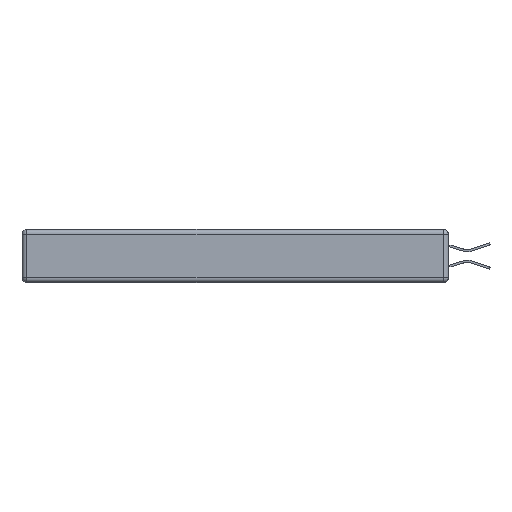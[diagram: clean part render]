
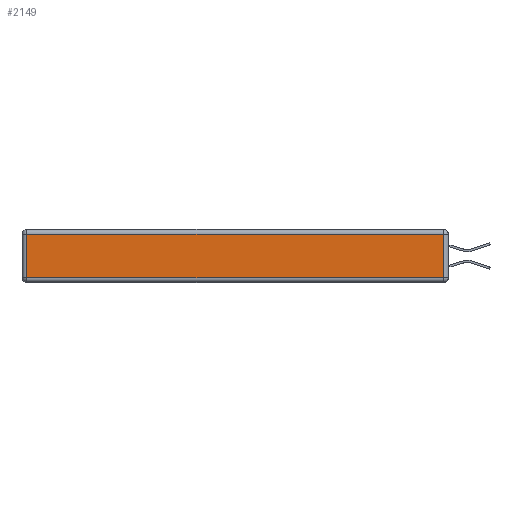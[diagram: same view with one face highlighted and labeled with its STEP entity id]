
A CAD part, left-side view. The second image highlights one B-rep face of the part: STEP entity #2149.
In plain terms, the highlighted planar face has unit normal (-1, 0, 0).
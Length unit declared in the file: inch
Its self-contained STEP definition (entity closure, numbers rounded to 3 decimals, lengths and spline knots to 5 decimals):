
#1864 = CARTESIAN_POINT ( 'NONE',  ( 0., 0.03, -0.313 ) ) ;
#2149 = ADVANCED_FACE ( 'NONE', ( #4905 ), #20034, .T. ) ;
#3078 = ORIENTED_EDGE ( 'NONE', *, *, #6674, .T. ) ;
#3151 = DIRECTION ( 'NONE',  ( 0., -1., 0. ) ) ;
#3313 = ORIENTED_EDGE ( 'NONE', *, *, #14853, .T. ) ;
#3814 = CARTESIAN_POINT ( 'NONE',  ( 0., 0.03, -0.03 ) ) ;
#4117 = EDGE_CURVE ( 'NONE', #13962, #17894, #7898, .T. ) ;
#4905 = FACE_OUTER_BOUND ( 'NONE', #19387, .T. ) ;
#5021 = LINE ( 'NONE', #6496, #16435 ) ;
#5069 = VERTEX_POINT ( 'NONE', #1864 ) ;
#6496 = CARTESIAN_POINT ( 'NONE',  ( 0., 2.75, -0.03 ) ) ;
#6674 = EDGE_CURVE ( 'NONE', #5069, #9211, #19468, .T. ) ;
#6957 = DIRECTION ( 'NONE',  ( 0., 0., 1. ) ) ;
#7348 = CARTESIAN_POINT ( 'NONE',  ( 0., 0., -0.313 ) ) ;
#7644 = ORIENTED_EDGE ( 'NONE', *, *, #12017, .T. ) ;
#7898 = LINE ( 'NONE', #18437, #13747 ) ;
#8716 = CARTESIAN_POINT ( 'NONE',  ( 0., 0.03, -0.343 ) ) ;
#9211 = VERTEX_POINT ( 'NONE', #3814 ) ;
#9344 = LINE ( 'NONE', #7348, #20005 ) ;
#9859 = DIRECTION ( 'NONE',  ( 0., 1., 0. ) ) ;
#10023 = CARTESIAN_POINT ( 'NONE',  ( 0., 2.72, -0.03 ) ) ;
#10199 = DIRECTION ( 'NONE',  ( -1., 0., 0. ) ) ;
#12017 = EDGE_CURVE ( 'NONE', #17894, #5069, #9344, .T. ) ;
#13747 = VECTOR ( 'NONE', #17927, 39.37008 ) ;
#13962 = VERTEX_POINT ( 'NONE', #10023 ) ;
#14397 = DIRECTION ( 'NONE',  ( 0., 0., 1. ) ) ;
#14853 = EDGE_CURVE ( 'NONE', #9211, #13962, #5021, .T. ) ;
#14999 = CARTESIAN_POINT ( 'NONE',  ( 0., 0., -0.343 ) ) ;
#15554 = AXIS2_PLACEMENT_3D ( 'NONE', #14999, #10199, #6957 ) ;
#16435 = VECTOR ( 'NONE', #9859, 39.37008 ) ;
#16465 = ORIENTED_EDGE ( 'NONE', *, *, #4117, .T. ) ;
#17894 = VERTEX_POINT ( 'NONE', #18928 ) ;
#17927 = DIRECTION ( 'NONE',  ( 0., 0., -1. ) ) ;
#18437 = CARTESIAN_POINT ( 'NONE',  ( 0., 2.72, -0.343 ) ) ;
#18928 = CARTESIAN_POINT ( 'NONE',  ( 0., 2.72, -0.313 ) ) ;
#19387 = EDGE_LOOP ( 'NONE', ( #7644, #3078, #3313, #16465 ) ) ;
#19468 = LINE ( 'NONE', #8716, #19998 ) ;
#19998 = VECTOR ( 'NONE', #14397, 39.37008 ) ;
#20005 = VECTOR ( 'NONE', #3151, 39.37008 ) ;
#20034 = PLANE ( 'NONE',  #15554 ) ;
